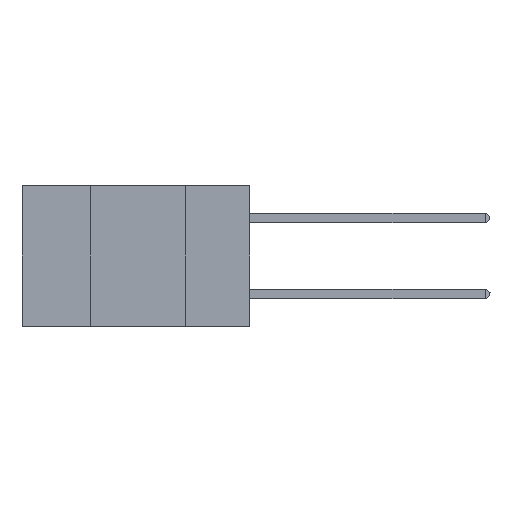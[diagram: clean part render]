
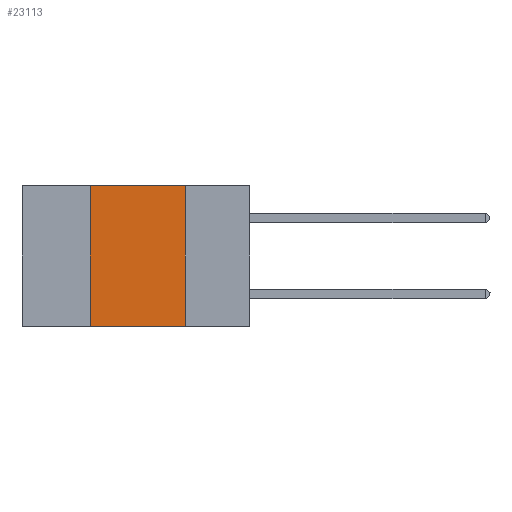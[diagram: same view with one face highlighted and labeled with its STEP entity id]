
A CAD part, left-side view. The second image highlights one B-rep face of the part: STEP entity #23113.
In plain terms, the highlighted planar face has unit normal (-1, 0, 0).
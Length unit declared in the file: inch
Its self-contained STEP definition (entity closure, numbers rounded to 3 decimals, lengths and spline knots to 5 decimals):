
#269 = ORIENTED_EDGE ( 'NONE', *, *, #22801, .F. ) ;
#2181 = EDGE_CURVE ( 'NONE', #20830, #15351, #21331, .T. ) ;
#2365 = LINE ( 'NONE', #26974, #26019 ) ;
#2378 = EDGE_CURVE ( 'NONE', #15469, #20830, #9172, .T. ) ;
#2486 = EDGE_CURVE ( 'NONE', #15469, #21131, #18777, .T. ) ;
#2540 = ORIENTED_EDGE ( 'NONE', *, *, #2486, .T. ) ;
#6620 = VECTOR ( 'NONE', #26597, 39.37008 ) ;
#8688 = CARTESIAN_POINT ( 'NONE',  ( 0., 0.17, 0. ) ) ;
#9172 = LINE ( 'NONE', #11865, #21675 ) ;
#9599 = DIRECTION ( 'NONE',  ( 0., 0., 1. ) ) ;
#10247 = VECTOR ( 'NONE', #13480, 39.37008 ) ;
#11167 = CARTESIAN_POINT ( 'NONE',  ( 0., 0.6, 0. ) ) ;
#11865 = CARTESIAN_POINT ( 'NONE',  ( 0., 0.42, 0. ) ) ;
#12938 = ORIENTED_EDGE ( 'NONE', *, *, #2181, .F. ) ;
#13480 = DIRECTION ( 'NONE',  ( 0., -1., 0. ) ) ;
#15351 = VERTEX_POINT ( 'NONE', #8688 ) ;
#15469 = VERTEX_POINT ( 'NONE', #26694 ) ;
#16722 = EDGE_LOOP ( 'NONE', ( #269, #12938, #20106, #2540 ) ) ;
#16893 = CARTESIAN_POINT ( 'NONE',  ( 0., 0.6, 0. ) ) ;
#16993 = DIRECTION ( 'NONE',  ( 0., 0., -1. ) ) ;
#17651 = CARTESIAN_POINT ( 'NONE',  ( 0., 0.6, -0.37 ) ) ;
#18777 = LINE ( 'NONE', #17651, #6620 ) ;
#19298 = CARTESIAN_POINT ( 'NONE',  ( 0., 0.17, -0.37 ) ) ;
#20106 = ORIENTED_EDGE ( 'NONE', *, *, #2378, .F. ) ;
#20439 = DIRECTION ( 'NONE',  ( 0., 0., -1. ) ) ;
#20830 = VERTEX_POINT ( 'NONE', #27559 ) ;
#21131 = VERTEX_POINT ( 'NONE', #19298 ) ;
#21331 = LINE ( 'NONE', #11167, #10247 ) ;
#21675 = VECTOR ( 'NONE', #9599, 39.37008 ) ;
#22801 = EDGE_CURVE ( 'NONE', #15351, #21131, #2365, .T. ) ;
#23113 = ADVANCED_FACE ( 'NONE', ( #25297 ), #26135, .F. ) ;
#25297 = FACE_OUTER_BOUND ( 'NONE', #16722, .T. ) ;
#26019 = VECTOR ( 'NONE', #20439, 39.37008 ) ;
#26135 = PLANE ( 'NONE',  #27988 ) ;
#26329 = DIRECTION ( 'NONE',  ( 1., 0., 0. ) ) ;
#26597 = DIRECTION ( 'NONE',  ( 0., -1., 0. ) ) ;
#26694 = CARTESIAN_POINT ( 'NONE',  ( 0., 0.42, -0.37 ) ) ;
#26974 = CARTESIAN_POINT ( 'NONE',  ( 0., 0.17, 0. ) ) ;
#27559 = CARTESIAN_POINT ( 'NONE',  ( 0., 0.42, 0. ) ) ;
#27988 = AXIS2_PLACEMENT_3D ( 'NONE', #16893, #26329, #16993 ) ;
